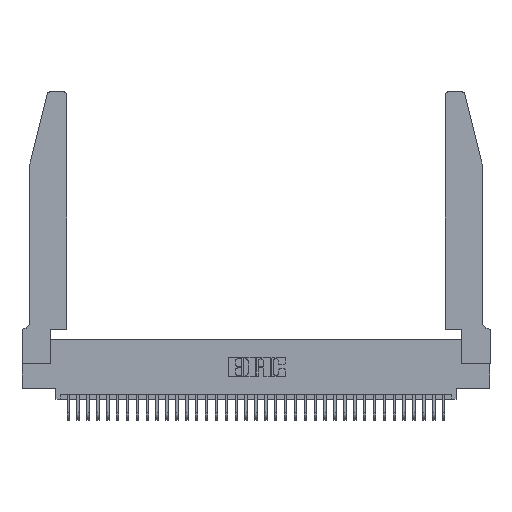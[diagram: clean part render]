
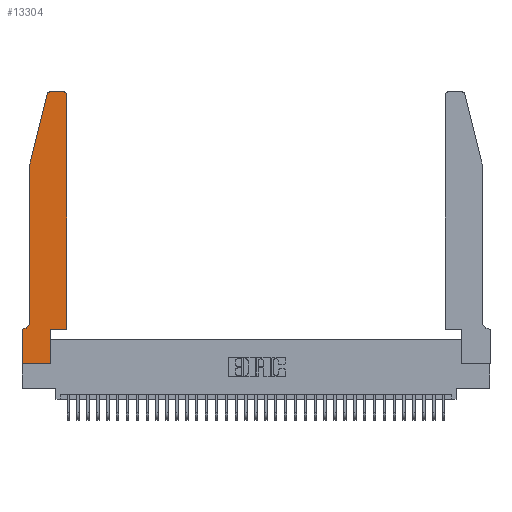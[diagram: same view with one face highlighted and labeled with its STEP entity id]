
A CAD part, top view. The second image highlights one B-rep face of the part: STEP entity #13304.
In plain terms, the highlighted planar face has unit normal (0, 0, 1).
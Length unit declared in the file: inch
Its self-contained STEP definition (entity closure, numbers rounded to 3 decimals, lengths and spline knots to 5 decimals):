
#221 = CARTESIAN_POINT ( 'NONE',  ( 0.4505, 2.72, 0.37 ) ) ;
#358 = ORIENTED_EDGE ( 'NONE', *, *, #13564, .T. ) ;
#510 = EDGE_CURVE ( 'NONE', #33713, #18578, #8063, .T. ) ;
#2949 = CARTESIAN_POINT ( 'NONE',  ( 0.0755, 2., 0.37 ) ) ;
#4093 = ORIENTED_EDGE ( 'NONE', *, *, #17339, .T. ) ;
#4626 = ORIENTED_EDGE ( 'NONE', *, *, #28880, .T. ) ;
#4828 = ORIENTED_EDGE ( 'NONE', *, *, #10456, .T. ) ;
#5458 = VERTEX_POINT ( 'NONE', #2949 ) ;
#5545 = CARTESIAN_POINT ( 'NONE',  ( 0.284, 2.72, 0.37 ) ) ;
#5630 = CARTESIAN_POINT ( 'NONE',  ( 0.0755, 0.35, 0.37 ) ) ;
#6029 = DIRECTION ( 'NONE',  ( 0., 0., 1. ) ) ;
#6647 = CARTESIAN_POINT ( 'NONE',  ( 0.2605, 2.75, 0.37 ) ) ;
#6954 = CARTESIAN_POINT ( 'NONE',  ( 0.4505, 0.35, 0.37 ) ) ;
#8041 = ORIENTED_EDGE ( 'NONE', *, *, #36621, .T. ) ;
#8063 = CIRCLE ( 'NONE', #17262, 0.03 ) ;
#8534 = DIRECTION ( 'NONE',  ( 1., 0., 0. ) ) ;
#9154 = CARTESIAN_POINT ( 'NONE',  ( 0.2865, 0.35, 0.37 ) ) ;
#9564 = LINE ( 'NONE', #5630, #16463 ) ;
#9653 = EDGE_CURVE ( 'NONE', #11299, #35229, #28207, .T. ) ;
#9950 = DIRECTION ( 'NONE',  ( 0., 1., 0. ) ) ;
#10057 = VECTOR ( 'NONE', #36090, 39.37008 ) ;
#10456 = EDGE_CURVE ( 'NONE', #16427, #25310, #9564, .T. ) ;
#11000 = DIRECTION ( 'NONE',  ( 0., -1., 0. ) ) ;
#11299 = VERTEX_POINT ( 'NONE', #29437 ) ;
#11593 = DIRECTION ( 'NONE',  ( -1., 0., 0. ) ) ;
#11801 = VECTOR ( 'NONE', #15297, 39.37008 ) ;
#12500 = DIRECTION ( 'NONE',  ( -1., 0., 0. ) ) ;
#12681 = ORIENTED_EDGE ( 'NONE', *, *, #12950, .T. ) ;
#12690 = VECTOR ( 'NONE', #9950, 39.37008 ) ;
#12765 = AXIS2_PLACEMENT_3D ( 'NONE', #32114, #14933, #34985 ) ;
#12849 = LINE ( 'NONE', #21699, #10057 ) ;
#12950 = EDGE_CURVE ( 'NONE', #35055, #33713, #19510, .T. ) ;
#13304 = ADVANCED_FACE ( 'NONE', ( #21256 ), #29138, .T. ) ;
#13445 = EDGE_CURVE ( 'NONE', #35229, #5458, #17668, .T. ) ;
#13564 = EDGE_CURVE ( 'NONE', #33543, #18982, #29294, .T. ) ;
#14190 = CARTESIAN_POINT ( 'NONE',  ( 0., 0., 0.37 ) ) ;
#14567 = CARTESIAN_POINT ( 'NONE',  ( 0.0055, 0.35, 0.37 ) ) ;
#14660 = ORIENTED_EDGE ( 'NONE', *, *, #37549, .T. ) ;
#14933 = DIRECTION ( 'NONE',  ( 0., 0., -1. ) ) ;
#15297 = DIRECTION ( 'NONE',  ( 0., 1., 0. ) ) ;
#16427 = VERTEX_POINT ( 'NONE', #14567 ) ;
#16463 = VECTOR ( 'NONE', #11593, 39.37008 ) ;
#16918 = CARTESIAN_POINT ( 'NONE',  ( 0.25487, 2.72718, 0.37 ) ) ;
#17262 = AXIS2_PLACEMENT_3D ( 'NONE', #22766, #33387, #33271 ) ;
#17339 = EDGE_CURVE ( 'NONE', #5458, #17874, #27737, .T. ) ;
#17668 = LINE ( 'NONE', #32513, #32866 ) ;
#17874 = VERTEX_POINT ( 'NONE', #25510 ) ;
#18238 = DIRECTION ( 'NONE',  ( -0.239, -0.971, 0. ) ) ;
#18578 = VERTEX_POINT ( 'NONE', #19927 ) ;
#18982 = VERTEX_POINT ( 'NONE', #31045 ) ;
#19510 = LINE ( 'NONE', #6954, #12690 ) ;
#19927 = CARTESIAN_POINT ( 'NONE',  ( 0.4205, 2.75, 0.37 ) ) ;
#20031 = LINE ( 'NONE', #33922, #26743 ) ;
#20120 = VECTOR ( 'NONE', #31664, 39.37008 ) ;
#21256 = FACE_OUTER_BOUND ( 'NONE', #24904, .T. ) ;
#21698 = VECTOR ( 'NONE', #30117, 39.37008 ) ;
#21699 = CARTESIAN_POINT ( 'NONE',  ( 0.4505, 0.35, 0.37 ) ) ;
#21808 = VERTEX_POINT ( 'NONE', #9154 ) ;
#22120 = ORIENTED_EDGE ( 'NONE', *, *, #510, .T. ) ;
#22766 = CARTESIAN_POINT ( 'NONE',  ( 0.4205, 2.72, 0.37 ) ) ;
#22942 = LINE ( 'NONE', #6647, #37266 ) ;
#24904 = EDGE_LOOP ( 'NONE', ( #29787, #26229, #33260, #4093, #31658, #4828, #8041, #358, #14660, #4626, #12681, #22120 ) ) ;
#25310 = VERTEX_POINT ( 'NONE', #32649 ) ;
#25510 = CARTESIAN_POINT ( 'NONE',  ( 0.0755, 0.42, 0.37 ) ) ;
#25943 = DIRECTION ( 'NONE',  ( 0., 0., 1. ) ) ;
#26229 = ORIENTED_EDGE ( 'NONE', *, *, #9653, .T. ) ;
#26402 = DIRECTION ( 'NONE',  ( 1., 0., 0. ) ) ;
#26743 = VECTOR ( 'NONE', #11000, 39.37008 ) ;
#26848 = CARTESIAN_POINT ( 'NONE',  ( 0.2865, 0.35, 0.37 ) ) ;
#27077 = CARTESIAN_POINT ( 'NONE',  ( 0.4505, 0.35, 0.37 ) ) ;
#27139 = EDGE_CURVE ( 'NONE', #18578, #11299, #22942, .T. ) ;
#27169 = LINE ( 'NONE', #26848, #11801 ) ;
#27737 = LINE ( 'NONE', #34399, #20120 ) ;
#28207 = CIRCLE ( 'NONE', #34584, 0.03 ) ;
#28880 = EDGE_CURVE ( 'NONE', #21808, #35055, #12849, .T. ) ;
#29138 = PLANE ( 'NONE',  #33200 ) ;
#29294 = LINE ( 'NONE', #29997, #21698 ) ;
#29437 = CARTESIAN_POINT ( 'NONE',  ( 0.284, 2.75, 0.37 ) ) ;
#29787 = ORIENTED_EDGE ( 'NONE', *, *, #27139, .T. ) ;
#29997 = CARTESIAN_POINT ( 'NONE',  ( 0., 0., 0.37 ) ) ;
#30117 = DIRECTION ( 'NONE',  ( 1., 0., 0. ) ) ;
#30754 = CIRCLE ( 'NONE', #12765, 0.07 ) ;
#31045 = CARTESIAN_POINT ( 'NONE',  ( 0.2865, 0., 0.37 ) ) ;
#31658 = ORIENTED_EDGE ( 'NONE', *, *, #37446, .T. ) ;
#31664 = DIRECTION ( 'NONE',  ( 0., -1., 0. ) ) ;
#32114 = CARTESIAN_POINT ( 'NONE',  ( 0.0055, 0.42, 0.37 ) ) ;
#32513 = CARTESIAN_POINT ( 'NONE',  ( 0.0755, 2., 0.37 ) ) ;
#32649 = CARTESIAN_POINT ( 'NONE',  ( 0., 0.35, 0.37 ) ) ;
#32866 = VECTOR ( 'NONE', #18238, 39.37008 ) ;
#33200 = AXIS2_PLACEMENT_3D ( 'NONE', #34770, #6029, #26402 ) ;
#33260 = ORIENTED_EDGE ( 'NONE', *, *, #13445, .T. ) ;
#33271 = DIRECTION ( 'NONE',  ( 1., 0., 0. ) ) ;
#33387 = DIRECTION ( 'NONE',  ( 0., 0., 1. ) ) ;
#33543 = VERTEX_POINT ( 'NONE', #14190 ) ;
#33713 = VERTEX_POINT ( 'NONE', #221 ) ;
#33922 = CARTESIAN_POINT ( 'NONE',  ( 0., 0., 0.37 ) ) ;
#34399 = CARTESIAN_POINT ( 'NONE',  ( 0.0755, 2., 0.37 ) ) ;
#34584 = AXIS2_PLACEMENT_3D ( 'NONE', #5545, #25943, #8534 ) ;
#34770 = CARTESIAN_POINT ( 'NONE',  ( 0., 0.35, 0.37 ) ) ;
#34985 = DIRECTION ( 'NONE',  ( -1., 0., 0. ) ) ;
#35055 = VERTEX_POINT ( 'NONE', #27077 ) ;
#35229 = VERTEX_POINT ( 'NONE', #16918 ) ;
#36090 = DIRECTION ( 'NONE',  ( 1., 0., 0. ) ) ;
#36621 = EDGE_CURVE ( 'NONE', #25310, #33543, #20031, .T. ) ;
#37266 = VECTOR ( 'NONE', #12500, 39.37008 ) ;
#37446 = EDGE_CURVE ( 'NONE', #17874, #16427, #30754, .T. ) ;
#37549 = EDGE_CURVE ( 'NONE', #18982, #21808, #27169, .T. ) ;
